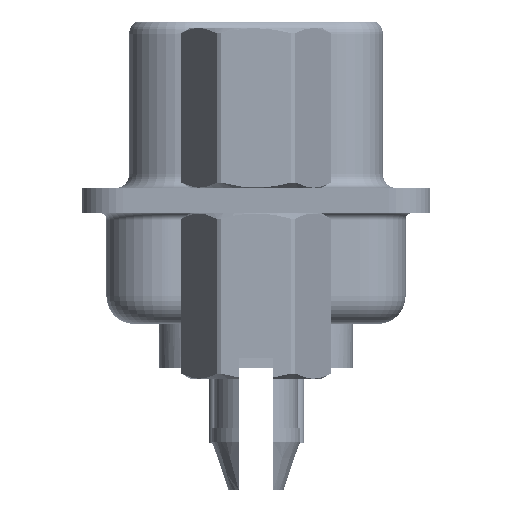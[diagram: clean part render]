
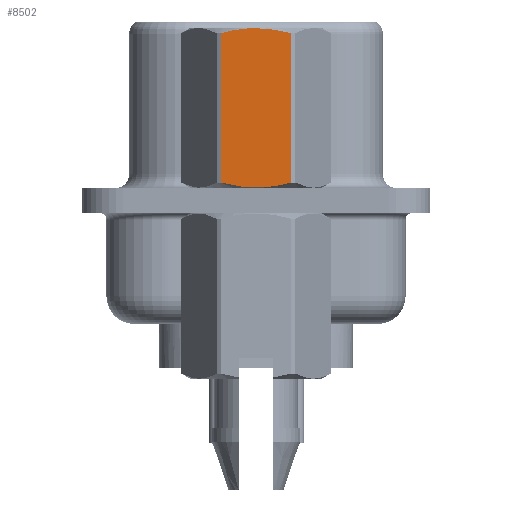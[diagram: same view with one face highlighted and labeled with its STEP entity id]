
A CAD part, left-side view. The second image highlights one B-rep face of the part: STEP entity #8502.
In plain terms, the highlighted planar face has unit normal (-1, 0, 0).
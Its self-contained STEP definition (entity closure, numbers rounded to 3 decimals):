
#1412 = CARTESIAN_POINT ( 'NONE',  ( -2.381, -0.432, 6.215 ) ) ;
#1909 = CARTESIAN_POINT ( 'NONE',  ( -2.381, 0.215, 0.468 ) ) ;
#4180 = CARTESIAN_POINT ( 'NONE',  ( -2.381, 1.375, -3.75 ) ) ;
#4200 = CARTESIAN_POINT ( 'NONE',  ( -2.381, 0.215, 6.232 ) ) ;
#4562 = CARTESIAN_POINT ( 'NONE',  ( -2.381, 1.273, 0.652 ) ) ;
#4679 = CARTESIAN_POINT ( 'NONE',  ( -2.381, -0.432, 0.485 ) ) ;
#5495 = CARTESIAN_POINT ( 'NONE',  ( -2.381, -1.273, 3.792 ) ) ;
#6958 = CARTESIAN_POINT ( 'NONE',  ( -2.381, 0.853, 6.151 ) ) ;
#7079 = CARTESIAN_POINT ( 'NONE',  ( -2.381, -1.273, 0.652 ) ) ;
#7428 = CARTESIAN_POINT ( 'NONE',  ( -2.381, -1.066, 0.596 ) ) ;
#8238 = DIRECTION ( 'NONE',  ( 0., 0., 1. ) ) ;
#8502 = ADVANCED_FACE ( 'NONE', ( #24589 ), #17860, .T. ) ;
#8573 = ORIENTED_EDGE ( 'NONE', *, *, #25361, .T. ) ;
#9581 = CARTESIAN_POINT ( 'NONE',  ( -2.381, -1.273, 6.048 ) ) ;
#9719 = CARTESIAN_POINT ( 'NONE',  ( -2.381, 1.273, 6.048 ) ) ;
#10875 = EDGE_CURVE ( 'NONE', #19472, #25908, #29754, .T. ) ;
#12470 = DIRECTION ( 'NONE',  ( 0., -1., 0. ) ) ;
#15106 = CARTESIAN_POINT ( 'NONE',  ( -2.381, 1.273, 3.792 ) ) ;
#15314 = AXIS2_PLACEMENT_3D ( 'NONE', #4180, #28838, #12470 ) ;
#15590 = CARTESIAN_POINT ( 'NONE',  ( -2.381, 0.853, 0.549 ) ) ;
#16580 = B_SPLINE_CURVE_WITH_KNOTS ( 'NONE', 3,
 ( #9581, #31437, #17876, #1412, #20609, #4200, #23362, #6958, #26130, #9719 ),
 .UNSPECIFIED., .F., .F.,
 ( 4, 2, 2, 2, 4 ),
 ( 0.001, 0.002, 0.002, 0.003, 0.004 ),
 .UNSPECIFIED. ) ;
#17293 = VECTOR ( 'NONE', #8238, 1000. ) ;
#17860 = PLANE ( 'NONE',  #15314 ) ;
#17876 = CARTESIAN_POINT ( 'NONE',  ( -2.381, -0.858, 6.15 ) ) ;
#18163 = LINE ( 'NONE', #5495, #17293 ) ;
#18359 = CARTESIAN_POINT ( 'NONE',  ( -2.381, 0.428, 0.485 ) ) ;
#19129 = EDGE_LOOP ( 'NONE', ( #30164, #8573, #27173, #32475 ) ) ;
#19472 = VERTEX_POINT ( 'NONE', #25054 ) ;
#19607 = CARTESIAN_POINT ( 'NONE',  ( -2.381, 1.273, 6.048 ) ) ;
#20609 = CARTESIAN_POINT ( 'NONE',  ( -2.381, -0.215, 6.232 ) ) ;
#21098 = CARTESIAN_POINT ( 'NONE',  ( -2.381, -0.215, 0.468 ) ) ;
#23362 = CARTESIAN_POINT ( 'NONE',  ( -2.381, 0.428, 6.215 ) ) ;
#23729 = CARTESIAN_POINT ( 'NONE',  ( -2.381, 1.065, 0.596 ) ) ;
#23856 = CARTESIAN_POINT ( 'NONE',  ( -2.381, -0.858, 0.55 ) ) ;
#24589 = FACE_OUTER_BOUND ( 'NONE', #19129, .T. ) ;
#25054 = CARTESIAN_POINT ( 'NONE',  ( -2.381, 1.273, 0.652 ) ) ;
#25361 = EDGE_CURVE ( 'NONE', #25908, #33955, #18163, .T. ) ;
#25846 = EDGE_CURVE ( 'NONE', #32682, #19472, #33447, .T. ) ;
#25908 = VERTEX_POINT ( 'NONE', #7079 ) ;
#26130 = CARTESIAN_POINT ( 'NONE',  ( -2.381, 1.065, 6.104 ) ) ;
#26605 = CARTESIAN_POINT ( 'NONE',  ( -2.381, -1.273, 0.652 ) ) ;
#27173 = ORIENTED_EDGE ( 'NONE', *, *, #35103, .T. ) ;
#28753 = DIRECTION ( 'NONE',  ( 0., 0., -1. ) ) ;
#28838 = DIRECTION ( 'NONE',  ( -1., 0., 0. ) ) ;
#29754 = B_SPLINE_CURVE_WITH_KNOTS ( 'NONE', 3,
 ( #4562, #23729, #15590, #18359, #1909, #21098, #4679, #23856, #7428, #26605 ),
 .UNSPECIFIED., .F., .F.,
 ( 4, 2, 2, 2, 4 ),
 ( 0.003, 0.003, 0.004, 0.004, 0.005 ),
 .UNSPECIFIED. ) ;
#30164 = ORIENTED_EDGE ( 'NONE', *, *, #10875, .T. ) ;
#31383 = CARTESIAN_POINT ( 'NONE',  ( -2.381, -1.273, 6.048 ) ) ;
#31437 = CARTESIAN_POINT ( 'NONE',  ( -2.381, -1.066, 6.104 ) ) ;
#32475 = ORIENTED_EDGE ( 'NONE', *, *, #25846, .T. ) ;
#32682 = VERTEX_POINT ( 'NONE', #19607 ) ;
#33447 = LINE ( 'NONE', #15106, #34315 ) ;
#33955 = VERTEX_POINT ( 'NONE', #31383 ) ;
#34315 = VECTOR ( 'NONE', #28753, 1000. ) ;
#35103 = EDGE_CURVE ( 'NONE', #33955, #32682, #16580, .T. ) ;
